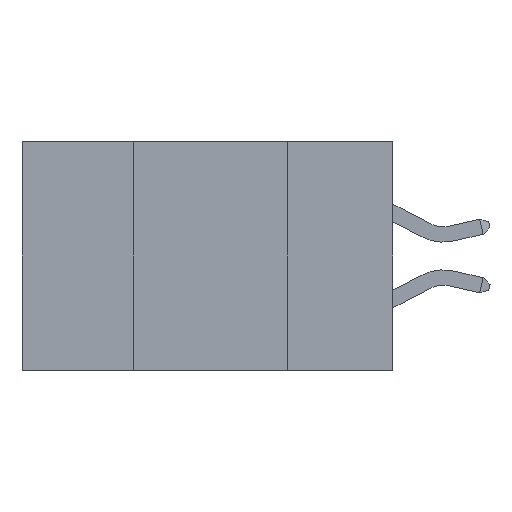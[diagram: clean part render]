
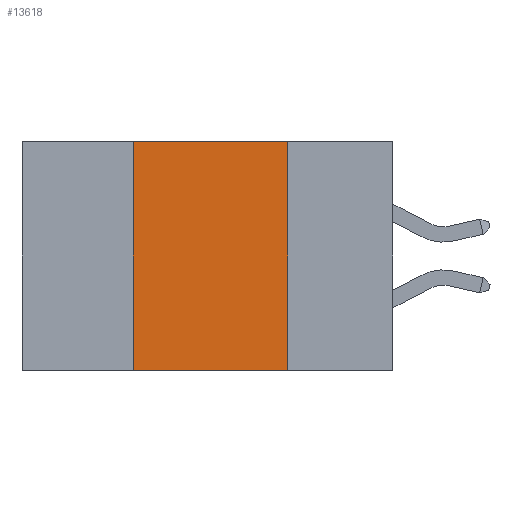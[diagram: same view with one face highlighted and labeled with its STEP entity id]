
A CAD part, left-side view. The second image highlights one B-rep face of the part: STEP entity #13618.
In plain terms, the highlighted planar face has unit normal (-1, 0, 0).
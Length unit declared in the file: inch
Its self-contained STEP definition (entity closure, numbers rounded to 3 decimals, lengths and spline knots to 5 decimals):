
#52 = ORIENTED_EDGE ( 'NONE', *, *, #12804, .F. ) ;
#873 = VECTOR ( 'NONE', #5067, 39.37008 ) ;
#1308 = EDGE_CURVE ( 'NONE', #7939, #18683, #7553, .T. ) ;
#1470 = ORIENTED_EDGE ( 'NONE', *, *, #13920, .F. ) ;
#2171 = LINE ( 'NONE', #10484, #3648 ) ;
#2444 = PLANE ( 'NONE',  #14842 ) ;
#3401 = CARTESIAN_POINT ( 'NONE',  ( 0., 0.6, 0. ) ) ;
#3648 = VECTOR ( 'NONE', #15424, 39.37008 ) ;
#4918 = EDGE_LOOP ( 'NONE', ( #1470, #52, #5266, #19184 ) ) ;
#5067 = DIRECTION ( 'NONE',  ( 0., -1., 0. ) ) ;
#5266 = ORIENTED_EDGE ( 'NONE', *, *, #1308, .F. ) ;
#7553 = LINE ( 'NONE', #16718, #15204 ) ;
#7939 = VERTEX_POINT ( 'NONE', #9156 ) ;
#8248 = DIRECTION ( 'NONE',  ( 0., 0., -1. ) ) ;
#8700 = FACE_OUTER_BOUND ( 'NONE', #4918, .T. ) ;
#9156 = CARTESIAN_POINT ( 'NONE',  ( 0., 0.42, -0.37 ) ) ;
#10484 = CARTESIAN_POINT ( 'NONE',  ( 0., 0.6, -0.37 ) ) ;
#10749 = CARTESIAN_POINT ( 'NONE',  ( 0., 0.17, 0. ) ) ;
#11133 = VERTEX_POINT ( 'NONE', #11443 ) ;
#11443 = CARTESIAN_POINT ( 'NONE',  ( 0., 0.17, -0.37 ) ) ;
#11893 = VECTOR ( 'NONE', #8248, 39.37008 ) ;
#12242 = CARTESIAN_POINT ( 'NONE',  ( 0., 0.42, 0. ) ) ;
#12804 = EDGE_CURVE ( 'NONE', #18683, #15057, #12897, .T. ) ;
#12897 = LINE ( 'NONE', #3401, #873 ) ;
#13449 = DIRECTION ( 'NONE',  ( 0., 0., -1. ) ) ;
#13618 = ADVANCED_FACE ( 'NONE', ( #8700 ), #2444, .F. ) ;
#13920 = EDGE_CURVE ( 'NONE', #15057, #11133, #16064, .T. ) ;
#14842 = AXIS2_PLACEMENT_3D ( 'NONE', #19833, #16446, #13449 ) ;
#15057 = VERTEX_POINT ( 'NONE', #10749 ) ;
#15204 = VECTOR ( 'NONE', #18236, 39.37008 ) ;
#15424 = DIRECTION ( 'NONE',  ( 0., -1., 0. ) ) ;
#16064 = LINE ( 'NONE', #17787, #11893 ) ;
#16446 = DIRECTION ( 'NONE',  ( 1., 0., 0. ) ) ;
#16718 = CARTESIAN_POINT ( 'NONE',  ( 0., 0.42, 0. ) ) ;
#17787 = CARTESIAN_POINT ( 'NONE',  ( 0., 0.17, 0. ) ) ;
#18234 = EDGE_CURVE ( 'NONE', #7939, #11133, #2171, .T. ) ;
#18236 = DIRECTION ( 'NONE',  ( 0., 0., 1. ) ) ;
#18683 = VERTEX_POINT ( 'NONE', #12242 ) ;
#19184 = ORIENTED_EDGE ( 'NONE', *, *, #18234, .T. ) ;
#19833 = CARTESIAN_POINT ( 'NONE',  ( 0., 0.6, 0. ) ) ;
